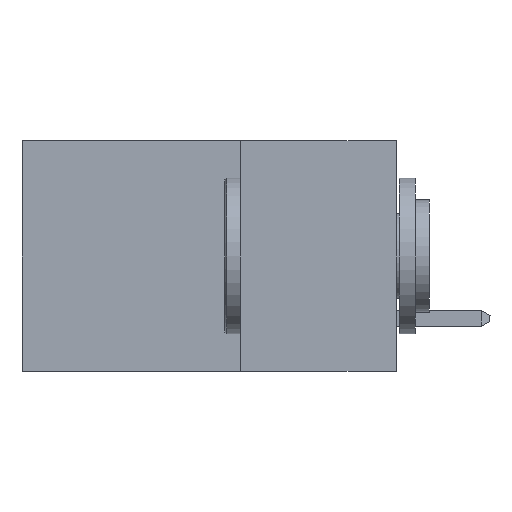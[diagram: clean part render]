
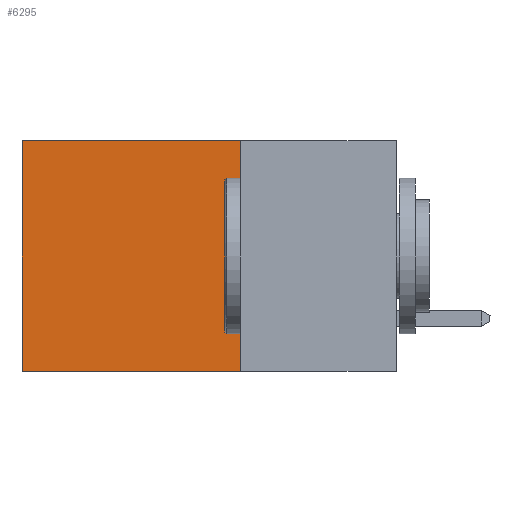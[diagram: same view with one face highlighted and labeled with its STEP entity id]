
A CAD part, left-side view. The second image highlights one B-rep face of the part: STEP entity #6295.
In plain terms, the highlighted planar face has unit normal (-1, 0, 0).
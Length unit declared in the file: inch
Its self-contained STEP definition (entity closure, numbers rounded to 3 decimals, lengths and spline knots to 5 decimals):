
#48 = CARTESIAN_POINT ( 'NONE',  ( 0.2615, 0.25, -0.37 ) ) ;
#290 = CARTESIAN_POINT ( 'NONE',  ( 0.2615, 0.6, -0.37 ) ) ;
#376 = DIRECTION ( 'NONE',  ( 0., 1., 0. ) ) ;
#824 = VERTEX_POINT ( 'NONE', #4542 ) ;
#1408 = ORIENTED_EDGE ( 'NONE', *, *, #5768, .F. ) ;
#1510 = AXIS2_PLACEMENT_3D ( 'NONE', #48, #4381, #2198 ) ;
#1815 = LINE ( 'NONE', #3403, #4611 ) ;
#2198 = DIRECTION ( 'NONE',  ( 0., 0., -1. ) ) ;
#2236 = VECTOR ( 'NONE', #6591, 39.37008 ) ;
#2268 = ORIENTED_EDGE ( 'NONE', *, *, #6524, .T. ) ;
#2387 = EDGE_CURVE ( 'NONE', #9342, #8192, #8744, .T. ) ;
#2429 = VECTOR ( 'NONE', #3524, 39.37008 ) ;
#2721 = CARTESIAN_POINT ( 'NONE',  ( 0.2615, 0.6, -0.37 ) ) ;
#2883 = FACE_OUTER_BOUND ( 'NONE', #8154, .T. ) ;
#3393 = DIRECTION ( 'NONE',  ( 0., 0., -1. ) ) ;
#3403 = CARTESIAN_POINT ( 'NONE',  ( 0.2615, 0.25, 0. ) ) ;
#3524 = DIRECTION ( 'NONE',  ( 0., 1., 0. ) ) ;
#3737 = EDGE_CURVE ( 'NONE', #824, #4266, #5293, .T. ) ;
#4266 = VERTEX_POINT ( 'NONE', #7578 ) ;
#4381 = DIRECTION ( 'NONE',  ( 1., 0., 0. ) ) ;
#4542 = CARTESIAN_POINT ( 'NONE',  ( 0.2615, 0.25, 0. ) ) ;
#4611 = VECTOR ( 'NONE', #376, 39.37008 ) ;
#5246 = ORIENTED_EDGE ( 'NONE', *, *, #2387, .T. ) ;
#5293 = LINE ( 'NONE', #7495, #2236 ) ;
#5768 = EDGE_CURVE ( 'NONE', #4266, #8192, #7907, .T. ) ;
#6295 = ADVANCED_FACE ( 'NONE', ( #2883 ), #8849, .F. ) ;
#6524 = EDGE_CURVE ( 'NONE', #824, #9342, #1815, .T. ) ;
#6591 = DIRECTION ( 'NONE',  ( 0., 0., -1. ) ) ;
#7097 = CARTESIAN_POINT ( 'NONE',  ( 0.2615, 0.25, -0.37 ) ) ;
#7495 = CARTESIAN_POINT ( 'NONE',  ( 0.2615, 0.25, -0.37 ) ) ;
#7578 = CARTESIAN_POINT ( 'NONE',  ( 0.2615, 0.25, -0.37 ) ) ;
#7907 = LINE ( 'NONE', #7097, #2429 ) ;
#8154 = EDGE_LOOP ( 'NONE', ( #5246, #1408, #9431, #2268 ) ) ;
#8192 = VERTEX_POINT ( 'NONE', #290 ) ;
#8725 = CARTESIAN_POINT ( 'NONE',  ( 0.2615, 0.6, 0. ) ) ;
#8744 = LINE ( 'NONE', #2721, #8829 ) ;
#8829 = VECTOR ( 'NONE', #3393, 39.37008 ) ;
#8849 = PLANE ( 'NONE',  #1510 ) ;
#9342 = VERTEX_POINT ( 'NONE', #8725 ) ;
#9431 = ORIENTED_EDGE ( 'NONE', *, *, #3737, .F. ) ;
